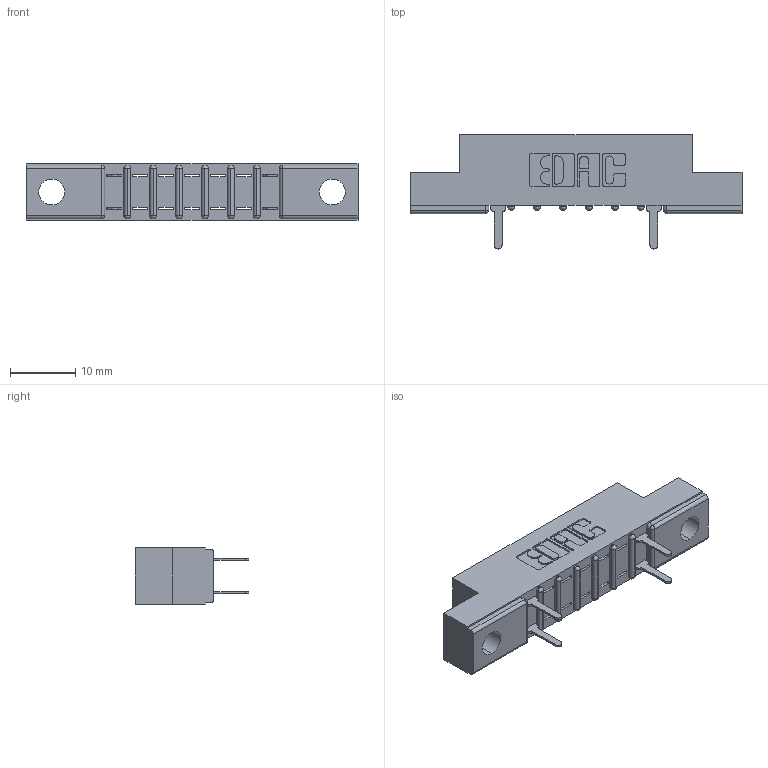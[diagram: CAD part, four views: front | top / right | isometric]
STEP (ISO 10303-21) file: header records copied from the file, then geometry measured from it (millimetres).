
FILE_DESCRIPTION (( 'STEP AP203' ), '1' );
FILE_NAME ('307-014-520-204.STEP', '2018-08-03T01:09:46', ( '' ), ( '' ), 'SwSTEP 2.0', 'SolidWorks 2016', '' );
FILE_SCHEMA (( 'CONFIG_CONTROL_DESIGN' ));
Length unit declared in the file: inch
Products named in the file (3): 307 Part_.156 Dia Mounting Holes; 307-290-001_520; 307-014-520-204
Assembly tree (5 placements, depth 2):
  307-014-520-204
    307 Part_.156 Dia Mounting Holes
    307-290-001_520  x4
Bounding box: 50.75 x 17.42 x 8.71 mm (x, y, z)
Volume: 3088.7 mm3; surface area: 3808.1 mm2
Topology: 5 solids, 5 shells, 424 faces, 1199 edges, 770 vertices
Faces by surface type: plane 268, cylinder 140, sphere 16
Entity records: 10606 total; most frequent: CARTESIAN_POINT 1791, ORIENTED_EDGE 1778, DIRECTION 1751, EDGE_CURVE 889, LINE 675, VECTOR 675, VERTEX_POINT 578, AXIS2_PLACEMENT_3D 538
